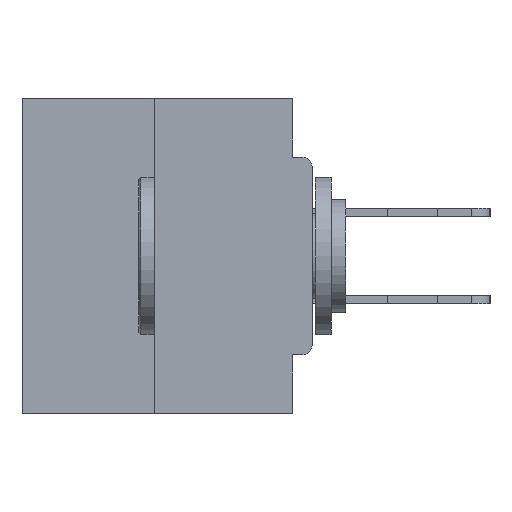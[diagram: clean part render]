
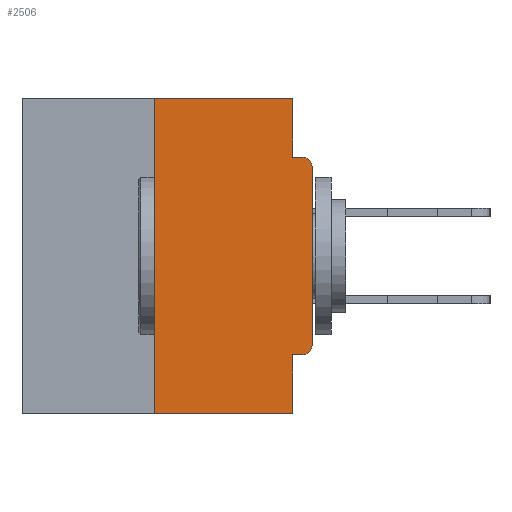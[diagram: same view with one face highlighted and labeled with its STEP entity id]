
A CAD part, left-side view. The second image highlights one B-rep face of the part: STEP entity #2506.
In plain terms, the highlighted planar face has unit normal (-1, 0, 0).
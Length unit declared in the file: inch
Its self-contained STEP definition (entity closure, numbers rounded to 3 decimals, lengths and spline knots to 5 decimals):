
#142 = CARTESIAN_POINT ( 'NONE',  ( 0., 0.031, 0. ) ) ;
#1482 = LINE ( 'NONE', #36750, #40279 ) ;
#2211 = CARTESIAN_POINT ( 'NONE',  ( 0., 0., -0.0935 ) ) ;
#2506 = ADVANCED_FACE ( 'NONE', ( #41347 ), #12548, .F. ) ;
#3635 = DIRECTION ( 'NONE',  ( 0., 0., -1. ) ) ;
#3947 = CARTESIAN_POINT ( 'NONE',  ( 0., 0.015, -0.3915 ) ) ;
#4198 = CARTESIAN_POINT ( 'NONE',  ( 0., 0.25, -0.5 ) ) ;
#4989 = DIRECTION ( 'NONE',  ( 0., 0., -1. ) ) ;
#5228 = CARTESIAN_POINT ( 'NONE',  ( 0., 0.031, -0.0935 ) ) ;
#5291 = LINE ( 'NONE', #23337, #15581 ) ;
#5336 = ORIENTED_EDGE ( 'NONE', *, *, #26160, .F. ) ;
#6219 = EDGE_LOOP ( 'NONE', ( #31346, #24265, #16546, #32957, #27453, #13608, #13306, #30975, #21965, #5336 ) ) ;
#6904 = VECTOR ( 'NONE', #3635, 39.37008 ) ;
#10539 = CARTESIAN_POINT ( 'NONE',  ( 0., 0.031, 0. ) ) ;
#12241 = DIRECTION ( 'NONE',  ( 1., 0., 0. ) ) ;
#12540 = DIRECTION ( 'NONE',  ( 0., -1., 0. ) ) ;
#12548 = PLANE ( 'NONE',  #26994 ) ;
#13306 = ORIENTED_EDGE ( 'NONE', *, *, #27658, .T. ) ;
#13457 = CARTESIAN_POINT ( 'NONE',  ( 0., 0.46, 0. ) ) ;
#13608 = ORIENTED_EDGE ( 'NONE', *, *, #33858, .T. ) ;
#14237 = CIRCLE ( 'NONE', #17363, 0.015 ) ;
#14834 = DIRECTION ( 'NONE',  ( -1., 0., 0. ) ) ;
#15581 = VECTOR ( 'NONE', #26815, 39.37008 ) ;
#15642 = CARTESIAN_POINT ( 'NONE',  ( 0., 0.015, -0.1085 ) ) ;
#16372 = VECTOR ( 'NONE', #34342, 39.37008 ) ;
#16546 = ORIENTED_EDGE ( 'NONE', *, *, #17042, .T. ) ;
#16562 = EDGE_CURVE ( 'NONE', #44274, #30186, #5291, .T. ) ;
#16798 = CARTESIAN_POINT ( 'NONE',  ( 0., 0., -0.1085 ) ) ;
#17042 = EDGE_CURVE ( 'NONE', #44274, #39002, #1482, .T. ) ;
#17363 = AXIS2_PLACEMENT_3D ( 'NONE', #15642, #40312, #26008 ) ;
#17675 = CARTESIAN_POINT ( 'NONE',  ( 0., 0.031, -0.5 ) ) ;
#18274 = LINE ( 'NONE', #17675, #6904 ) ;
#19987 = CIRCLE ( 'NONE', #20916, 0.015 ) ;
#20786 = CARTESIAN_POINT ( 'NONE',  ( 0., 0.015, -0.4065 ) ) ;
#20916 = AXIS2_PLACEMENT_3D ( 'NONE', #3947, #14834, #25072 ) ;
#21475 = CARTESIAN_POINT ( 'NONE',  ( 0., 0.031, -0.5 ) ) ;
#21912 = CARTESIAN_POINT ( 'NONE',  ( 0., 0., -0.3915 ) ) ;
#21965 = ORIENTED_EDGE ( 'NONE', *, *, #22530, .F. ) ;
#22530 = EDGE_CURVE ( 'NONE', #27779, #32523, #39186, .T. ) ;
#23337 = CARTESIAN_POINT ( 'NONE',  ( 0., 0.25, 0. ) ) ;
#23541 = VECTOR ( 'NONE', #28900, 39.37008 ) ;
#24145 = VECTOR ( 'NONE', #37061, 39.37008 ) ;
#24265 = ORIENTED_EDGE ( 'NONE', *, *, #16562, .F. ) ;
#24809 = VECTOR ( 'NONE', #27419, 39.37008 ) ;
#24933 = VERTEX_POINT ( 'NONE', #35418 ) ;
#25072 = DIRECTION ( 'NONE',  ( 0., 0., -1. ) ) ;
#25136 = EDGE_CURVE ( 'NONE', #30186, #26255, #28744, .T. ) ;
#26008 = DIRECTION ( 'NONE',  ( 0., 0., -1. ) ) ;
#26160 = EDGE_CURVE ( 'NONE', #26255, #27779, #43088, .T. ) ;
#26255 = VERTEX_POINT ( 'NONE', #142 ) ;
#26815 = DIRECTION ( 'NONE',  ( 0., 0., 1. ) ) ;
#26994 = AXIS2_PLACEMENT_3D ( 'NONE', #32830, #12241, #4989 ) ;
#27161 = EDGE_CURVE ( 'NONE', #24933, #39002, #18274, .T. ) ;
#27419 = DIRECTION ( 'NONE',  ( 0., 0., -1. ) ) ;
#27453 = ORIENTED_EDGE ( 'NONE', *, *, #44410, .F. ) ;
#27658 = EDGE_CURVE ( 'NONE', #43554, #35545, #44566, .T. ) ;
#27779 = VERTEX_POINT ( 'NONE', #5228 ) ;
#28294 = VERTEX_POINT ( 'NONE', #20786 ) ;
#28384 = VECTOR ( 'NONE', #42578, 39.37008 ) ;
#28456 = LINE ( 'NONE', #43968, #24145 ) ;
#28744 = LINE ( 'NONE', #13457, #16372 ) ;
#28900 = DIRECTION ( 'NONE',  ( 0., 0., 1. ) ) ;
#30186 = VERTEX_POINT ( 'NONE', #37720 ) ;
#30975 = ORIENTED_EDGE ( 'NONE', *, *, #41269, .T. ) ;
#31346 = ORIENTED_EDGE ( 'NONE', *, *, #25136, .F. ) ;
#32037 = CARTESIAN_POINT ( 'NONE',  ( 0., 0., 0. ) ) ;
#32523 = VERTEX_POINT ( 'NONE', #34521 ) ;
#32830 = CARTESIAN_POINT ( 'NONE',  ( 0., 0.46, 0. ) ) ;
#32957 = ORIENTED_EDGE ( 'NONE', *, *, #27161, .F. ) ;
#33858 = EDGE_CURVE ( 'NONE', #28294, #43554, #19987, .T. ) ;
#34342 = DIRECTION ( 'NONE',  ( 0., -1., 0. ) ) ;
#34521 = CARTESIAN_POINT ( 'NONE',  ( 0., 0.015, -0.0935 ) ) ;
#35418 = CARTESIAN_POINT ( 'NONE',  ( 0., 0.031, -0.4065 ) ) ;
#35545 = VERTEX_POINT ( 'NONE', #16798 ) ;
#36750 = CARTESIAN_POINT ( 'NONE',  ( 0., 0.46, -0.5 ) ) ;
#37061 = DIRECTION ( 'NONE',  ( 0., 1., 0. ) ) ;
#37720 = CARTESIAN_POINT ( 'NONE',  ( 0., 0.25, 0. ) ) ;
#39002 = VERTEX_POINT ( 'NONE', #21475 ) ;
#39186 = LINE ( 'NONE', #2211, #28384 ) ;
#40279 = VECTOR ( 'NONE', #12540, 39.37008 ) ;
#40312 = DIRECTION ( 'NONE',  ( -1., 0., 0. ) ) ;
#41269 = EDGE_CURVE ( 'NONE', #35545, #32523, #14237, .T. ) ;
#41347 = FACE_OUTER_BOUND ( 'NONE', #6219, .T. ) ;
#42578 = DIRECTION ( 'NONE',  ( 0., -1., 0. ) ) ;
#43088 = LINE ( 'NONE', #10539, #24809 ) ;
#43554 = VERTEX_POINT ( 'NONE', #21912 ) ;
#43968 = CARTESIAN_POINT ( 'NONE',  ( 0., 0., -0.4065 ) ) ;
#44274 = VERTEX_POINT ( 'NONE', #4198 ) ;
#44410 = EDGE_CURVE ( 'NONE', #28294, #24933, #28456, .T. ) ;
#44566 = LINE ( 'NONE', #32037, #23541 ) ;
